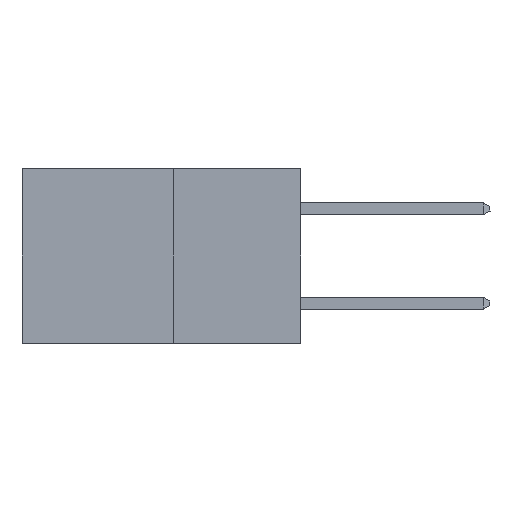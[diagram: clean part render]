
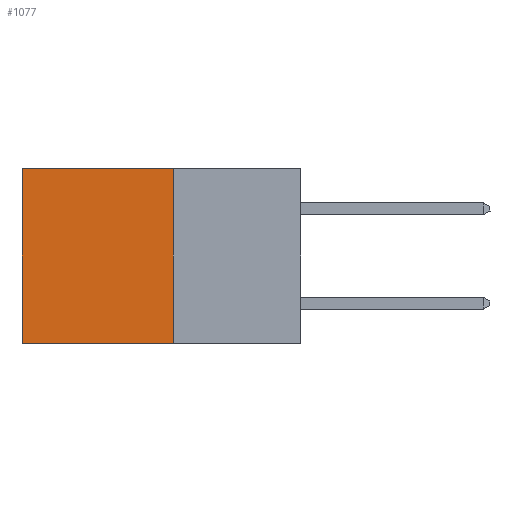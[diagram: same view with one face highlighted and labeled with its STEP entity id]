
A CAD part, left-side view. The second image highlights one B-rep face of the part: STEP entity #1077.
In plain terms, the highlighted planar face has unit normal (-1, 0, 0).
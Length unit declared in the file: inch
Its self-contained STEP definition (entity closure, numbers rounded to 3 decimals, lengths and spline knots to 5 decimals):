
#198 = CARTESIAN_POINT ( 'NONE',  ( 0.277, 0.27, 0. ) ) ;
#231 = ORIENTED_EDGE ( 'NONE', *, *, #5975, .F. ) ;
#477 = CARTESIAN_POINT ( 'NONE',  ( 0.277, 0.27, -0.37 ) ) ;
#557 = CARTESIAN_POINT ( 'NONE',  ( 0.277, 0.27, -0.37 ) ) ;
#667 = PLANE ( 'NONE',  #9098 ) ;
#908 = CARTESIAN_POINT ( 'NONE',  ( 0.277, 0.59, -0.37 ) ) ;
#1002 = VERTEX_POINT ( 'NONE', #908 ) ;
#1077 = ADVANCED_FACE ( 'NONE', ( #8231 ), #667, .F. ) ;
#1297 = CARTESIAN_POINT ( 'NONE',  ( 0.277, 0.27, -0.37 ) ) ;
#1487 = LINE ( 'NONE', #557, #9585 ) ;
#1613 = VERTEX_POINT ( 'NONE', #198 ) ;
#1679 = DIRECTION ( 'NONE',  ( 0., 0., -1. ) ) ;
#1868 = LINE ( 'NONE', #1297, #9693 ) ;
#1924 = DIRECTION ( 'NONE',  ( 1., 0., 0. ) ) ;
#1958 = CARTESIAN_POINT ( 'NONE',  ( 0.277, 0.27, 0. ) ) ;
#2143 = VERTEX_POINT ( 'NONE', #8020 ) ;
#4054 = CARTESIAN_POINT ( 'NONE',  ( 0.277, 0.59, -0.37 ) ) ;
#4186 = VECTOR ( 'NONE', #9534, 39.37008 ) ;
#4836 = EDGE_LOOP ( 'NONE', ( #7067, #4905, #231, #8117 ) ) ;
#4905 = ORIENTED_EDGE ( 'NONE', *, *, #9749, .F. ) ;
#5363 = CARTESIAN_POINT ( 'NONE',  ( 0.277, 0.59, 0. ) ) ;
#5834 = EDGE_CURVE ( 'NONE', #1613, #9119, #6192, .T. ) ;
#5975 = EDGE_CURVE ( 'NONE', #1613, #2143, #1868, .T. ) ;
#6136 = DIRECTION ( 'NONE',  ( 0., 1., 0. ) ) ;
#6192 = LINE ( 'NONE', #1958, #4186 ) ;
#7067 = ORIENTED_EDGE ( 'NONE', *, *, #8648, .T. ) ;
#7503 = DIRECTION ( 'NONE',  ( 0., 0., -1. ) ) ;
#8020 = CARTESIAN_POINT ( 'NONE',  ( 0.277, 0.27, -0.37 ) ) ;
#8043 = VECTOR ( 'NONE', #9920, 39.37008 ) ;
#8117 = ORIENTED_EDGE ( 'NONE', *, *, #5834, .T. ) ;
#8231 = FACE_OUTER_BOUND ( 'NONE', #4836, .T. ) ;
#8648 = EDGE_CURVE ( 'NONE', #9119, #1002, #9949, .T. ) ;
#9098 = AXIS2_PLACEMENT_3D ( 'NONE', #477, #1924, #1679 ) ;
#9119 = VERTEX_POINT ( 'NONE', #5363 ) ;
#9534 = DIRECTION ( 'NONE',  ( 0., 1., 0. ) ) ;
#9585 = VECTOR ( 'NONE', #6136, 39.37008 ) ;
#9693 = VECTOR ( 'NONE', #7503, 39.37008 ) ;
#9749 = EDGE_CURVE ( 'NONE', #2143, #1002, #1487, .T. ) ;
#9920 = DIRECTION ( 'NONE',  ( 0., 0., -1. ) ) ;
#9949 = LINE ( 'NONE', #4054, #8043 ) ;
